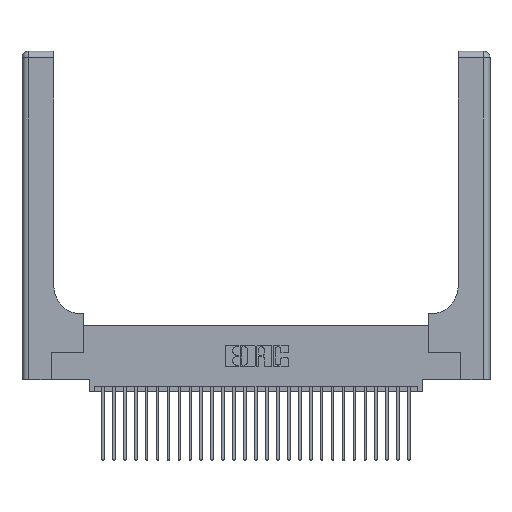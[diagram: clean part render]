
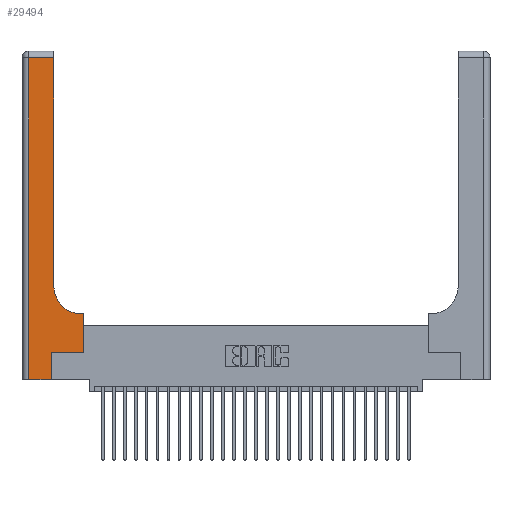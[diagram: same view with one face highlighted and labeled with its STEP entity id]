
A CAD part, top view. The second image highlights one B-rep face of the part: STEP entity #29494.
In plain terms, the highlighted planar face has unit normal (0, 0, 1).
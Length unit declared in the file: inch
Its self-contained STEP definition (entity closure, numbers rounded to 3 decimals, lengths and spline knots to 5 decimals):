
#1204 = DIRECTION ( 'NONE',  ( 0., 1., 0. ) ) ;
#2395 = CIRCLE ( 'NONE', #23862, 0.25 ) ;
#2697 = VERTEX_POINT ( 'NONE', #14208 ) ;
#2872 = LINE ( 'NONE', #11284, #14379 ) ;
#3559 = CARTESIAN_POINT ( 'NONE',  ( 0.5415, 0.85, 0.37 ) ) ;
#3801 = DIRECTION ( 'NONE',  ( 1., 0., 0. ) ) ;
#3994 = LINE ( 'NONE', #19519, #23129 ) ;
#4009 = CARTESIAN_POINT ( 'NONE',  ( 0., 0., 0.37 ) ) ;
#5449 = ORIENTED_EDGE ( 'NONE', *, *, #7938, .T. ) ;
#5822 = FACE_OUTER_BOUND ( 'NONE', #28013, .T. ) ;
#7010 = EDGE_CURVE ( 'NONE', #12745, #8389, #9376, .T. ) ;
#7361 = EDGE_CURVE ( 'NONE', #2697, #29269, #13678, .T. ) ;
#7938 = EDGE_CURVE ( 'NONE', #29269, #12745, #2872, .T. ) ;
#8106 = CARTESIAN_POINT ( 'NONE',  ( 0.2915, 0.6, 0.37 ) ) ;
#8389 = VERTEX_POINT ( 'NONE', #26291 ) ;
#8489 = PLANE ( 'NONE',  #14521 ) ;
#8788 = DIRECTION ( 'NONE',  ( 0., -1., 0. ) ) ;
#8968 = CARTESIAN_POINT ( 'NONE',  ( 0.5415, 0.6, 0.37 ) ) ;
#9020 = VECTOR ( 'NONE', #3801, 39.37008 ) ;
#9049 = DIRECTION ( 'NONE',  ( 1., 0., 0. ) ) ;
#9158 = EDGE_CURVE ( 'NONE', #11530, #27057, #21889, .T. ) ;
#9376 = LINE ( 'NONE', #10948, #18441 ) ;
#9522 = ORIENTED_EDGE ( 'NONE', *, *, #12755, .T. ) ;
#9992 = LINE ( 'NONE', #29712, #10706 ) ;
#10233 = CARTESIAN_POINT ( 'NONE',  ( 0.269, 0.25, 0.37 ) ) ;
#10676 = VECTOR ( 'NONE', #14412, 39.37008 ) ;
#10706 = VECTOR ( 'NONE', #8788, 39.37008 ) ;
#10948 = CARTESIAN_POINT ( 'NONE',  ( 0.269, 0.25, 0.37 ) ) ;
#11284 = CARTESIAN_POINT ( 'NONE',  ( 0.269, 0., 0.37 ) ) ;
#11530 = VERTEX_POINT ( 'NONE', #27702 ) ;
#12306 = CARTESIAN_POINT ( 'NONE',  ( 0.5585, 0.25, 0.37 ) ) ;
#12745 = VERTEX_POINT ( 'NONE', #10233 ) ;
#12755 = EDGE_CURVE ( 'NONE', #22538, #21477, #3994, .T. ) ;
#12835 = DIRECTION ( 'NONE',  ( -1., 0., 0. ) ) ;
#13182 = CARTESIAN_POINT ( 'NONE',  ( 0.2915, 2.94, 0.37 ) ) ;
#13678 = LINE ( 'NONE', #4009, #9020 ) ;
#14208 = CARTESIAN_POINT ( 'NONE',  ( 0.06, 0., 0.37 ) ) ;
#14379 = VECTOR ( 'NONE', #24914, 39.37008 ) ;
#14412 = DIRECTION ( 'NONE',  ( 0., 1., 0. ) ) ;
#14521 = AXIS2_PLACEMENT_3D ( 'NONE', #27049, #15551, #12835 ) ;
#14956 = CARTESIAN_POINT ( 'NONE',  ( 0.269, 0., 0.37 ) ) ;
#15551 = DIRECTION ( 'NONE',  ( 0., 0., -1. ) ) ;
#16303 = VECTOR ( 'NONE', #21201, 39.37008 ) ;
#17523 = VECTOR ( 'NONE', #24238, 39.37008 ) ;
#18101 = LINE ( 'NONE', #19188, #16303 ) ;
#18441 = VECTOR ( 'NONE', #9049, 39.37008 ) ;
#18762 = CARTESIAN_POINT ( 'NONE',  ( 0.06, 2.94, 0.37 ) ) ;
#19188 = CARTESIAN_POINT ( 'NONE',  ( 0., 2.94, 0.37 ) ) ;
#19394 = DIRECTION ( 'NONE',  ( 0., 0., -1. ) ) ;
#19451 = EDGE_CURVE ( 'NONE', #27057, #22538, #2395, .T. ) ;
#19519 = CARTESIAN_POINT ( 'NONE',  ( 0.2915, 3., 0.37 ) ) ;
#19687 = DIRECTION ( 'NONE',  ( 1., 0., 0. ) ) ;
#21019 = ORIENTED_EDGE ( 'NONE', *, *, #26327, .T. ) ;
#21201 = DIRECTION ( 'NONE',  ( -1., 0., 0. ) ) ;
#21477 = VERTEX_POINT ( 'NONE', #13182 ) ;
#21481 = ORIENTED_EDGE ( 'NONE', *, *, #7010, .T. ) ;
#21889 = LINE ( 'NONE', #8106, #17523 ) ;
#22181 = ORIENTED_EDGE ( 'NONE', *, *, #7361, .T. ) ;
#22538 = VERTEX_POINT ( 'NONE', #28272 ) ;
#22563 = EDGE_CURVE ( 'NONE', #21477, #25347, #18101, .T. ) ;
#23129 = VECTOR ( 'NONE', #1204, 39.37008 ) ;
#23862 = AXIS2_PLACEMENT_3D ( 'NONE', #3559, #19394, #19687 ) ;
#24238 = DIRECTION ( 'NONE',  ( -1., 0., 0. ) ) ;
#24575 = ORIENTED_EDGE ( 'NONE', *, *, #22563, .T. ) ;
#24890 = ORIENTED_EDGE ( 'NONE', *, *, #9158, .T. ) ;
#24914 = DIRECTION ( 'NONE',  ( 0., 1., 0. ) ) ;
#25347 = VERTEX_POINT ( 'NONE', #18762 ) ;
#25981 = ORIENTED_EDGE ( 'NONE', *, *, #19451, .T. ) ;
#26291 = CARTESIAN_POINT ( 'NONE',  ( 0.5585, 0.25, 0.37 ) ) ;
#26327 = EDGE_CURVE ( 'NONE', #25347, #2697, #9992, .T. ) ;
#26622 = EDGE_CURVE ( 'NONE', #8389, #11530, #29125, .T. ) ;
#27049 = CARTESIAN_POINT ( 'NONE',  ( 0., 3., 0.37 ) ) ;
#27057 = VERTEX_POINT ( 'NONE', #8968 ) ;
#27702 = CARTESIAN_POINT ( 'NONE',  ( 0.5585, 0.6, 0.37 ) ) ;
#27804 = ORIENTED_EDGE ( 'NONE', *, *, #26622, .T. ) ;
#28013 = EDGE_LOOP ( 'NONE', ( #9522, #24575, #21019, #22181, #5449, #21481, #27804, #24890, #25981 ) ) ;
#28272 = CARTESIAN_POINT ( 'NONE',  ( 0.2915, 0.85, 0.37 ) ) ;
#29125 = LINE ( 'NONE', #12306, #10676 ) ;
#29269 = VERTEX_POINT ( 'NONE', #14956 ) ;
#29494 = ADVANCED_FACE ( 'NONE', ( #5822 ), #8489, .F. ) ;
#29712 = CARTESIAN_POINT ( 'NONE',  ( 0.06, 3., 0.37 ) ) ;
